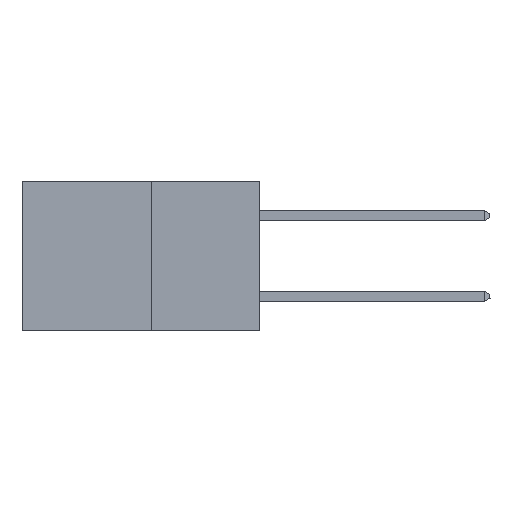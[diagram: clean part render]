
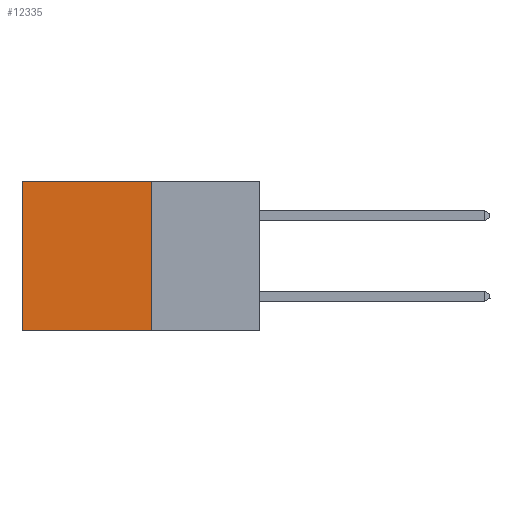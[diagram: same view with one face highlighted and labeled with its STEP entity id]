
A CAD part, left-side view. The second image highlights one B-rep face of the part: STEP entity #12335.
In plain terms, the highlighted planar face has unit normal (-1, 0, 0).
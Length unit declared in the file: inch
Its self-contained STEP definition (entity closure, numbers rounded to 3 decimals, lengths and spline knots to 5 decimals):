
#685 = VECTOR ( 'NONE', #15499, 39.37008 ) ;
#1239 = VERTEX_POINT ( 'NONE', #1657 ) ;
#1607 = CARTESIAN_POINT ( 'NONE',  ( 0.277, 0.27, 0. ) ) ;
#1657 = CARTESIAN_POINT ( 'NONE',  ( 0.277, 0.27, -0.37 ) ) ;
#3426 = EDGE_CURVE ( 'NONE', #1239, #12794, #4387, .T. ) ;
#4079 = EDGE_LOOP ( 'NONE', ( #9817, #17459, #14251, #19232 ) ) ;
#4387 = LINE ( 'NONE', #17824, #17550 ) ;
#5708 = VERTEX_POINT ( 'NONE', #15268 ) ;
#7000 = LINE ( 'NONE', #1607, #685 ) ;
#7042 = FACE_OUTER_BOUND ( 'NONE', #4079, .T. ) ;
#7092 = CARTESIAN_POINT ( 'NONE',  ( 0.277, 0.59, -0.37 ) ) ;
#8254 = DIRECTION ( 'NONE',  ( 0., 0., -1. ) ) ;
#8588 = LINE ( 'NONE', #13365, #21729 ) ;
#8829 = EDGE_CURVE ( 'NONE', #5708, #1239, #20297, .T. ) ;
#9817 = ORIENTED_EDGE ( 'NONE', *, *, #21564, .T. ) ;
#11073 = DIRECTION ( 'NONE',  ( 0., 1., 0. ) ) ;
#11169 = DIRECTION ( 'NONE',  ( 0., 0., -1. ) ) ;
#11172 = VECTOR ( 'NONE', #19434, 39.37008 ) ;
#11189 = DIRECTION ( 'NONE',  ( 1., 0., 0. ) ) ;
#11194 = CARTESIAN_POINT ( 'NONE',  ( 0.277, 0.27, -0.37 ) ) ;
#11216 = PLANE ( 'NONE',  #17600 ) ;
#12335 = ADVANCED_FACE ( 'NONE', ( #7042 ), #11216, .F. ) ;
#12794 = VERTEX_POINT ( 'NONE', #7092 ) ;
#13365 = CARTESIAN_POINT ( 'NONE',  ( 0.277, 0.59, -0.37 ) ) ;
#14251 = ORIENTED_EDGE ( 'NONE', *, *, #8829, .F. ) ;
#15268 = CARTESIAN_POINT ( 'NONE',  ( 0.277, 0.27, 0. ) ) ;
#15499 = DIRECTION ( 'NONE',  ( 0., 1., 0. ) ) ;
#16075 = EDGE_CURVE ( 'NONE', #5708, #22131, #7000, .T. ) ;
#17459 = ORIENTED_EDGE ( 'NONE', *, *, #3426, .F. ) ;
#17550 = VECTOR ( 'NONE', #11073, 39.37008 ) ;
#17600 = AXIS2_PLACEMENT_3D ( 'NONE', #11194, #11189, #11169 ) ;
#17824 = CARTESIAN_POINT ( 'NONE',  ( 0.277, 0.27, -0.37 ) ) ;
#19232 = ORIENTED_EDGE ( 'NONE', *, *, #16075, .T. ) ;
#19434 = DIRECTION ( 'NONE',  ( 0., 0., -1. ) ) ;
#19466 = CARTESIAN_POINT ( 'NONE',  ( 0.277, 0.27, -0.37 ) ) ;
#20297 = LINE ( 'NONE', #19466, #11172 ) ;
#21564 = EDGE_CURVE ( 'NONE', #22131, #12794, #8588, .T. ) ;
#21573 = CARTESIAN_POINT ( 'NONE',  ( 0.277, 0.59, 0. ) ) ;
#21729 = VECTOR ( 'NONE', #8254, 39.37008 ) ;
#22131 = VERTEX_POINT ( 'NONE', #21573 ) ;
